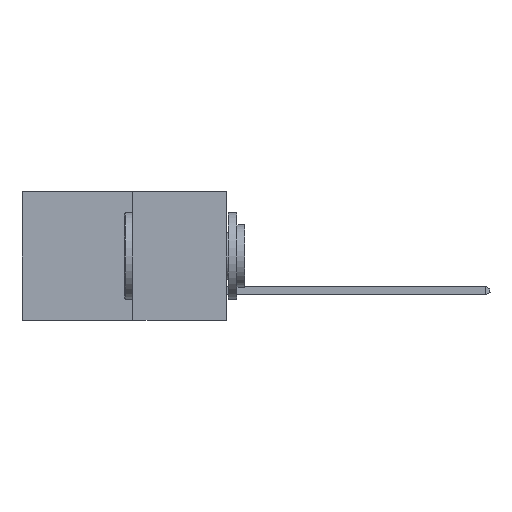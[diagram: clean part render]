
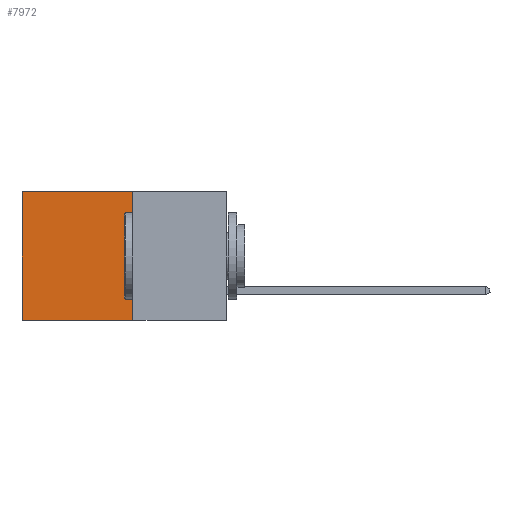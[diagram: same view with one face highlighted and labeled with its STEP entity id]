
A CAD part, left-side view. The second image highlights one B-rep face of the part: STEP entity #7972.
In plain terms, the highlighted planar face has unit normal (-1, 0, 0).
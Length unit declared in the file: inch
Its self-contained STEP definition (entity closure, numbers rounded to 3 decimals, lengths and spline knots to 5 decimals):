
#207 = EDGE_CURVE ( 'NONE', #6205, #6348, #10414, .T. ) ;
#437 = DIRECTION ( 'NONE',  ( 0., 1., 0. ) ) ;
#752 = CARTESIAN_POINT ( 'NONE',  ( 0.277, 0.59, 0. ) ) ;
#820 = VECTOR ( 'NONE', #12410, 39.37008 ) ;
#914 = CARTESIAN_POINT ( 'NONE',  ( 0.277, 0.27, 0. ) ) ;
#1164 = FACE_OUTER_BOUND ( 'NONE', #6853, .T. ) ;
#1216 = DIRECTION ( 'NONE',  ( 0., 0., -1. ) ) ;
#1221 = EDGE_CURVE ( 'NONE', #3954, #6205, #7805, .T. ) ;
#3477 = CARTESIAN_POINT ( 'NONE',  ( 0.277, 0.27, -0.37 ) ) ;
#3954 = VERTEX_POINT ( 'NONE', #10705 ) ;
#4790 = EDGE_CURVE ( 'NONE', #3954, #8853, #6801, .T. ) ;
#5174 = VECTOR ( 'NONE', #6778, 39.37008 ) ;
#5461 = DIRECTION ( 'NONE',  ( 0., 0., -1. ) ) ;
#5661 = VECTOR ( 'NONE', #5461, 39.37008 ) ;
#5888 = CARTESIAN_POINT ( 'NONE',  ( 0.277, 0.59, -0.37 ) ) ;
#6205 = VERTEX_POINT ( 'NONE', #12339 ) ;
#6348 = VERTEX_POINT ( 'NONE', #5888 ) ;
#6378 = ORIENTED_EDGE ( 'NONE', *, *, #7630, .T. ) ;
#6778 = DIRECTION ( 'NONE',  ( 0., 0., -1. ) ) ;
#6797 = CARTESIAN_POINT ( 'NONE',  ( 0.277, 0.27, -0.37 ) ) ;
#6801 = LINE ( 'NONE', #914, #820 ) ;
#6853 = EDGE_LOOP ( 'NONE', ( #6378, #10756, #9456, #12070 ) ) ;
#7630 = EDGE_CURVE ( 'NONE', #8853, #6348, #10859, .T. ) ;
#7762 = DIRECTION ( 'NONE',  ( 1., 0., 0. ) ) ;
#7805 = LINE ( 'NONE', #6797, #5174 ) ;
#7972 = ADVANCED_FACE ( 'NONE', ( #1164 ), #10620, .F. ) ;
#8478 = VECTOR ( 'NONE', #437, 39.37008 ) ;
#8853 = VERTEX_POINT ( 'NONE', #752 ) ;
#9456 = ORIENTED_EDGE ( 'NONE', *, *, #1221, .F. ) ;
#9480 = CARTESIAN_POINT ( 'NONE',  ( 0.277, 0.27, -0.37 ) ) ;
#10359 = AXIS2_PLACEMENT_3D ( 'NONE', #3477, #7762, #1216 ) ;
#10414 = LINE ( 'NONE', #9480, #8478 ) ;
#10620 = PLANE ( 'NONE',  #10359 ) ;
#10705 = CARTESIAN_POINT ( 'NONE',  ( 0.277, 0.27, 0. ) ) ;
#10756 = ORIENTED_EDGE ( 'NONE', *, *, #207, .F. ) ;
#10859 = LINE ( 'NONE', #12302, #5661 ) ;
#12070 = ORIENTED_EDGE ( 'NONE', *, *, #4790, .T. ) ;
#12302 = CARTESIAN_POINT ( 'NONE',  ( 0.277, 0.59, -0.37 ) ) ;
#12339 = CARTESIAN_POINT ( 'NONE',  ( 0.277, 0.27, -0.37 ) ) ;
#12410 = DIRECTION ( 'NONE',  ( 0., 1., 0. ) ) ;
